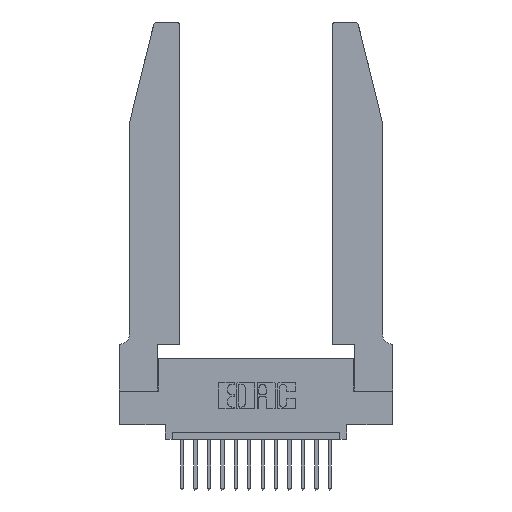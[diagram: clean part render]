
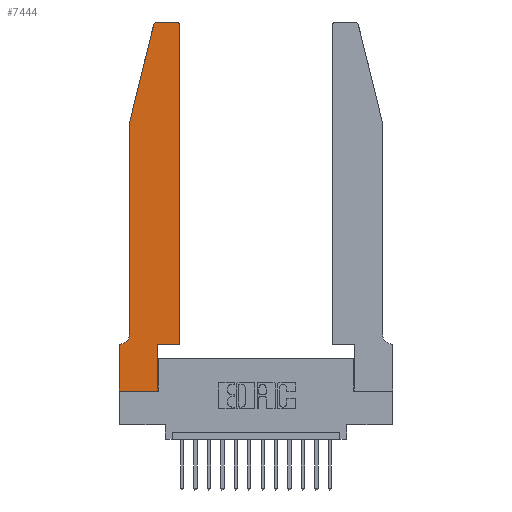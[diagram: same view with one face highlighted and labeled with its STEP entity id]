
A CAD part, top view. The second image highlights one B-rep face of the part: STEP entity #7444.
In plain terms, the highlighted planar face has unit normal (0, 0, 1).
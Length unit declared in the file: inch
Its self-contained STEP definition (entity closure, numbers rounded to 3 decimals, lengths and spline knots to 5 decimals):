
#161 = EDGE_CURVE ( 'NONE', #670, #14144, #7186, .T. ) ;
#174 = ORIENTED_EDGE ( 'NONE', *, *, #12933, .T. ) ;
#275 = CARTESIAN_POINT ( 'NONE',  ( 0.284, 2.72, 0.37 ) ) ;
#437 = DIRECTION ( 'NONE',  ( 0., 0., 1. ) ) ;
#641 = DIRECTION ( 'NONE',  ( 0., -1., 0. ) ) ;
#670 = VERTEX_POINT ( 'NONE', #13765 ) ;
#755 = DIRECTION ( 'NONE',  ( 0., -1., 0. ) ) ;
#818 = CARTESIAN_POINT ( 'NONE',  ( 0.4205, 2.75, 0.37 ) ) ;
#1421 = CARTESIAN_POINT ( 'NONE',  ( 0.4505, 0.35, 0.37 ) ) ;
#1701 = CARTESIAN_POINT ( 'NONE',  ( 0.2605, 2.75, 0.37 ) ) ;
#1835 = EDGE_CURVE ( 'NONE', #5401, #670, #11976, .T. ) ;
#2172 = CARTESIAN_POINT ( 'NONE',  ( 0.0755, 0.35, 0.37 ) ) ;
#2333 = VERTEX_POINT ( 'NONE', #818 ) ;
#2518 = CIRCLE ( 'NONE', #6789, 0.03 ) ;
#2707 = DIRECTION ( 'NONE',  ( 1., 0., 0. ) ) ;
#2860 = CARTESIAN_POINT ( 'NONE',  ( 0.0755, 2., 0.37 ) ) ;
#2891 = DIRECTION ( 'NONE',  ( 0., 1., 0. ) ) ;
#3026 = LINE ( 'NONE', #1701, #9507 ) ;
#3365 = CARTESIAN_POINT ( 'NONE',  ( 0.2865, 0.35, 0.37 ) ) ;
#3536 = ORIENTED_EDGE ( 'NONE', *, *, #6607, .T. ) ;
#3678 = EDGE_CURVE ( 'NONE', #7927, #17721, #5414, .T. ) ;
#4318 = ORIENTED_EDGE ( 'NONE', *, *, #7631, .T. ) ;
#4501 = EDGE_CURVE ( 'NONE', #2333, #4664, #3026, .T. ) ;
#4664 = VERTEX_POINT ( 'NONE', #16258 ) ;
#5052 = DIRECTION ( 'NONE',  ( 0., 0., 1. ) ) ;
#5401 = VERTEX_POINT ( 'NONE', #5438 ) ;
#5414 = LINE ( 'NONE', #2860, #5614 ) ;
#5438 = CARTESIAN_POINT ( 'NONE',  ( 0.0055, 0.35, 0.37 ) ) ;
#5614 = VECTOR ( 'NONE', #12686, 39.37008 ) ;
#5686 = ORIENTED_EDGE ( 'NONE', *, *, #6701, .T. ) ;
#6276 = LINE ( 'NONE', #9038, #13675 ) ;
#6607 = EDGE_CURVE ( 'NONE', #11136, #5401, #9886, .T. ) ;
#6701 = EDGE_CURVE ( 'NONE', #10307, #2333, #2518, .T. ) ;
#6789 = AXIS2_PLACEMENT_3D ( 'NONE', #15896, #437, #11807 ) ;
#6821 = CARTESIAN_POINT ( 'NONE',  ( 0.2865, 0., 0.37 ) ) ;
#6994 = CARTESIAN_POINT ( 'NONE',  ( 0.25487, 2.72718, 0.37 ) ) ;
#7085 = ORIENTED_EDGE ( 'NONE', *, *, #8875, .T. ) ;
#7089 = CARTESIAN_POINT ( 'NONE',  ( 0.4505, 0.35, 0.37 ) ) ;
#7098 = DIRECTION ( 'NONE',  ( 0., 0., 1. ) ) ;
#7186 = LINE ( 'NONE', #11835, #13050 ) ;
#7195 = DIRECTION ( 'NONE',  ( 1., 0., 0. ) ) ;
#7444 = ADVANCED_FACE ( 'NONE', ( #15488 ), #11143, .T. ) ;
#7515 = ORIENTED_EDGE ( 'NONE', *, *, #1835, .T. ) ;
#7608 = VECTOR ( 'NONE', #17761, 39.37008 ) ;
#7631 = EDGE_CURVE ( 'NONE', #16634, #11381, #12042, .T. ) ;
#7927 = VERTEX_POINT ( 'NONE', #6994 ) ;
#8027 = CIRCLE ( 'NONE', #13525, 0.03 ) ;
#8235 = VECTOR ( 'NONE', #13331, 39.37008 ) ;
#8310 = CARTESIAN_POINT ( 'NONE',  ( 0.4505, 2.72, 0.37 ) ) ;
#8875 = EDGE_CURVE ( 'NONE', #14144, #16303, #13268, .T. ) ;
#8968 = DIRECTION ( 'NONE',  ( 0., 0., -1. ) ) ;
#9038 = CARTESIAN_POINT ( 'NONE',  ( 0.0755, 2., 0.37 ) ) ;
#9507 = VECTOR ( 'NONE', #10129, 39.37008 ) ;
#9886 = CIRCLE ( 'NONE', #16676, 0.07 ) ;
#10129 = DIRECTION ( 'NONE',  ( -1., 0., 0. ) ) ;
#10183 = CARTESIAN_POINT ( 'NONE',  ( 0.4505, 0.35, 0.37 ) ) ;
#10204 = EDGE_LOOP ( 'NONE', ( #17813, #12868, #13710, #174, #3536, #7515, #17891, #7085, #14745, #4318, #15662, #5686 ) ) ;
#10307 = VERTEX_POINT ( 'NONE', #8310 ) ;
#10334 = DIRECTION ( 'NONE',  ( 0., 1., 0. ) ) ;
#11136 = VERTEX_POINT ( 'NONE', #16223 ) ;
#11143 = PLANE ( 'NONE',  #17153 ) ;
#11214 = CARTESIAN_POINT ( 'NONE',  ( 0., 0.35, 0.37 ) ) ;
#11381 = VERTEX_POINT ( 'NONE', #7089 ) ;
#11485 = CARTESIAN_POINT ( 'NONE',  ( 0.0755, 2., 0.37 ) ) ;
#11807 = DIRECTION ( 'NONE',  ( 1., 0., 0. ) ) ;
#11835 = CARTESIAN_POINT ( 'NONE',  ( 0., 0., 0.37 ) ) ;
#11976 = LINE ( 'NONE', #2172, #8235 ) ;
#12042 = LINE ( 'NONE', #10183, #13775 ) ;
#12417 = EDGE_CURVE ( 'NONE', #4664, #7927, #8027, .T. ) ;
#12434 = LINE ( 'NONE', #14558, #15658 ) ;
#12686 = DIRECTION ( 'NONE',  ( -0.239, -0.971, 0. ) ) ;
#12868 = ORIENTED_EDGE ( 'NONE', *, *, #12417, .T. ) ;
#12933 = EDGE_CURVE ( 'NONE', #17721, #11136, #6276, .T. ) ;
#13050 = VECTOR ( 'NONE', #641, 39.37008 ) ;
#13080 = LINE ( 'NONE', #1421, #14398 ) ;
#13268 = LINE ( 'NONE', #13760, #7608 ) ;
#13298 = DIRECTION ( 'NONE',  ( -1., 0., 0. ) ) ;
#13331 = DIRECTION ( 'NONE',  ( -1., 0., 0. ) ) ;
#13525 = AXIS2_PLACEMENT_3D ( 'NONE', #275, #5052, #17545 ) ;
#13675 = VECTOR ( 'NONE', #755, 39.37008 ) ;
#13710 = ORIENTED_EDGE ( 'NONE', *, *, #3678, .T. ) ;
#13760 = CARTESIAN_POINT ( 'NONE',  ( 0., 0., 0.37 ) ) ;
#13765 = CARTESIAN_POINT ( 'NONE',  ( 0., 0.35, 0.37 ) ) ;
#13775 = VECTOR ( 'NONE', #7195, 39.37008 ) ;
#14144 = VERTEX_POINT ( 'NONE', #17297 ) ;
#14398 = VECTOR ( 'NONE', #2891, 39.37008 ) ;
#14558 = CARTESIAN_POINT ( 'NONE',  ( 0.2865, 0.35, 0.37 ) ) ;
#14745 = ORIENTED_EDGE ( 'NONE', *, *, #17166, .T. ) ;
#15488 = FACE_OUTER_BOUND ( 'NONE', #10204, .T. ) ;
#15658 = VECTOR ( 'NONE', #10334, 39.37008 ) ;
#15662 = ORIENTED_EDGE ( 'NONE', *, *, #16433, .T. ) ;
#15896 = CARTESIAN_POINT ( 'NONE',  ( 0.4205, 2.72, 0.37 ) ) ;
#16223 = CARTESIAN_POINT ( 'NONE',  ( 0.0755, 0.42, 0.37 ) ) ;
#16258 = CARTESIAN_POINT ( 'NONE',  ( 0.284, 2.75, 0.37 ) ) ;
#16303 = VERTEX_POINT ( 'NONE', #6821 ) ;
#16433 = EDGE_CURVE ( 'NONE', #11381, #10307, #13080, .T. ) ;
#16634 = VERTEX_POINT ( 'NONE', #3365 ) ;
#16676 = AXIS2_PLACEMENT_3D ( 'NONE', #17413, #8968, #13298 ) ;
#17153 = AXIS2_PLACEMENT_3D ( 'NONE', #11214, #7098, #2707 ) ;
#17166 = EDGE_CURVE ( 'NONE', #16303, #16634, #12434, .T. ) ;
#17297 = CARTESIAN_POINT ( 'NONE',  ( 0., 0., 0.37 ) ) ;
#17413 = CARTESIAN_POINT ( 'NONE',  ( 0.0055, 0.42, 0.37 ) ) ;
#17545 = DIRECTION ( 'NONE',  ( 1., 0., 0. ) ) ;
#17721 = VERTEX_POINT ( 'NONE', #11485 ) ;
#17761 = DIRECTION ( 'NONE',  ( 1., 0., 0. ) ) ;
#17813 = ORIENTED_EDGE ( 'NONE', *, *, #4501, .T. ) ;
#17891 = ORIENTED_EDGE ( 'NONE', *, *, #161, .T. ) ;
